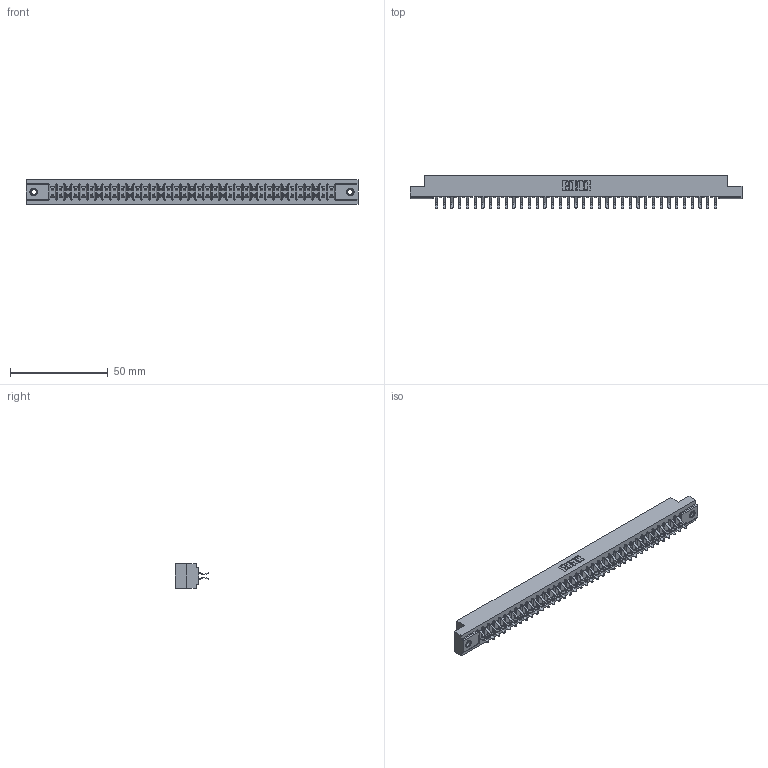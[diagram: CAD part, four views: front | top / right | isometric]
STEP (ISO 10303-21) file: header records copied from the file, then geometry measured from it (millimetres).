
FILE_DESCRIPTION (( 'STEP AP203' ), '1' );
FILE_NAME ('357-074-456-207.STEP', '2020-10-04T17:11:42', ( '' ), ( '' ), 'SwSTEP 2.0', 'SolidWorks 2020', '' );
FILE_SCHEMA (( 'CONFIG_CONTROL_DESIGN' ));
Length unit declared in the file: inch
Products named in the file (4): 345-250-001_345-250-005-103; 357-074-456-207; 307-290-001_556; 307 Part_.156 Dia Mounting Holes
Assembly tree (77 placements, depth 2):
  357-074-456-207
    307 Part_.156 Dia Mounting Holes
    307-290-001_556  x74
    345-250-001_345-250-005-103  x2
Bounding box: 169.62 x 16.97 x 12.7 mm (x, y, z)
Volume: 17974.8 mm3; surface area: 21730.7 mm2
Topology: 77 solids, 77 shells, 3916 faces, 10967 edges, 7102 vertices
Faces by surface type: plane 2544, cylinder 1280, sphere 76, cone 12, torus 4
Entity records: 34809 total; most frequent: CARTESIAN_POINT 5680, ORIENTED_EDGE 5622, DIRECTION 5575, EDGE_CURVE 2811, VECTOR 2153, LINE 2153, VERTEX_POINT 1816, AXIS2_PLACEMENT_3D 1711
